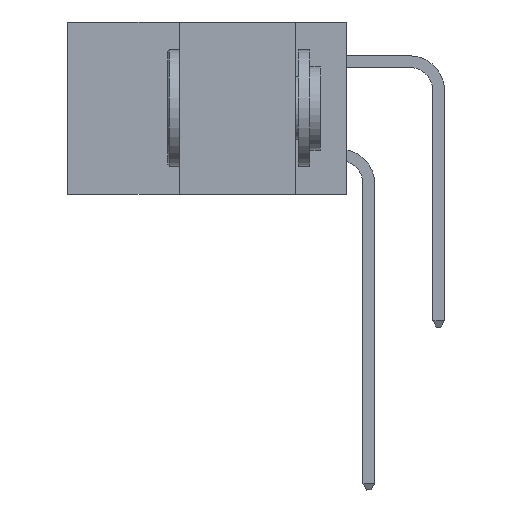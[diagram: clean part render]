
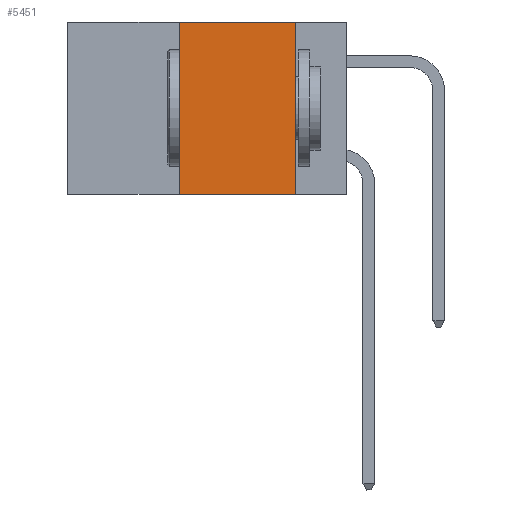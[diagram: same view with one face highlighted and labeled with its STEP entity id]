
A CAD part, left-side view. The second image highlights one B-rep face of the part: STEP entity #5451.
In plain terms, the highlighted planar face has unit normal (-1, 0, 0).
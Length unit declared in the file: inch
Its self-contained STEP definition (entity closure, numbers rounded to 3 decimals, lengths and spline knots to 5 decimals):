
#837 = VECTOR ( 'NONE', #3317, 39.37008 ) ;
#1083 = VERTEX_POINT ( 'NONE', #7972 ) ;
#1561 = DIRECTION ( 'NONE',  ( 0., -1., 0. ) ) ;
#2702 = VECTOR ( 'NONE', #1561, 39.37008 ) ;
#3216 = CARTESIAN_POINT ( 'NONE',  ( 0., 0.6, -0.37 ) ) ;
#3317 = DIRECTION ( 'NONE',  ( 0., -1., 0. ) ) ;
#3996 = VERTEX_POINT ( 'NONE', #24081 ) ;
#4937 = LINE ( 'NONE', #26119, #27395 ) ;
#5451 = ADVANCED_FACE ( 'NONE', ( #9324 ), #20472, .F. ) ;
#5578 = VERTEX_POINT ( 'NONE', #25266 ) ;
#5609 = ORIENTED_EDGE ( 'NONE', *, *, #12746, .F. ) ;
#7015 = ORIENTED_EDGE ( 'NONE', *, *, #14645, .F. ) ;
#7359 = DIRECTION ( 'NONE',  ( 1., 0., 0. ) ) ;
#7972 = CARTESIAN_POINT ( 'NONE',  ( 0., 0.11, -0.37 ) ) ;
#8658 = LINE ( 'NONE', #25497, #2702 ) ;
#8666 = EDGE_LOOP ( 'NONE', ( #5609, #7015, #15011, #21384 ) ) ;
#9324 = FACE_OUTER_BOUND ( 'NONE', #8666, .T. ) ;
#11783 = CARTESIAN_POINT ( 'NONE',  ( 0., 0.6, 0. ) ) ;
#12746 = EDGE_CURVE ( 'NONE', #25791, #1083, #4937, .T. ) ;
#14645 = EDGE_CURVE ( 'NONE', #5578, #25791, #8658, .T. ) ;
#15011 = ORIENTED_EDGE ( 'NONE', *, *, #25882, .F. ) ;
#15631 = VECTOR ( 'NONE', #25170, 39.37008 ) ;
#16309 = LINE ( 'NONE', #16553, #15631 ) ;
#16553 = CARTESIAN_POINT ( 'NONE',  ( 0., 0.36, 0. ) ) ;
#19125 = LINE ( 'NONE', #3216, #837 ) ;
#20102 = DIRECTION ( 'NONE',  ( 0., 0., -1. ) ) ;
#20472 = PLANE ( 'NONE',  #26749 ) ;
#20566 = CARTESIAN_POINT ( 'NONE',  ( 0., 0.11, 0. ) ) ;
#21384 = ORIENTED_EDGE ( 'NONE', *, *, #22104, .T. ) ;
#22104 = EDGE_CURVE ( 'NONE', #3996, #1083, #19125, .T. ) ;
#22637 = DIRECTION ( 'NONE',  ( 0., 0., -1. ) ) ;
#24081 = CARTESIAN_POINT ( 'NONE',  ( 0., 0.36, -0.37 ) ) ;
#25170 = DIRECTION ( 'NONE',  ( 0., 0., 1. ) ) ;
#25266 = CARTESIAN_POINT ( 'NONE',  ( 0., 0.36, 0. ) ) ;
#25497 = CARTESIAN_POINT ( 'NONE',  ( 0., 0.6, 0. ) ) ;
#25791 = VERTEX_POINT ( 'NONE', #20566 ) ;
#25882 = EDGE_CURVE ( 'NONE', #3996, #5578, #16309, .T. ) ;
#26119 = CARTESIAN_POINT ( 'NONE',  ( 0., 0.11, 0. ) ) ;
#26749 = AXIS2_PLACEMENT_3D ( 'NONE', #11783, #7359, #22637 ) ;
#27395 = VECTOR ( 'NONE', #20102, 39.37008 ) ;
